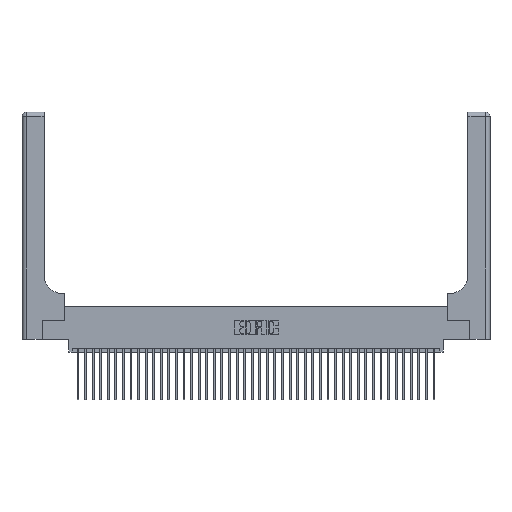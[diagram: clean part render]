
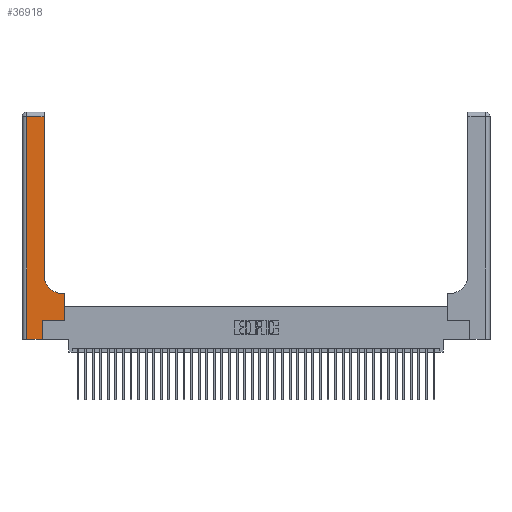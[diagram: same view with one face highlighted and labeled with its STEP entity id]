
A CAD part, top view. The second image highlights one B-rep face of the part: STEP entity #36918.
In plain terms, the highlighted planar face has unit normal (0, 0, 1).
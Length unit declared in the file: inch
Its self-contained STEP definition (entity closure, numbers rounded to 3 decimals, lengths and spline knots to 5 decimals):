
#201 = CARTESIAN_POINT ( 'NONE',  ( 0.2915, 0.85, 0.37 ) ) ;
#1006 = VECTOR ( 'NONE', #35913, 39.37008 ) ;
#1096 = DIRECTION ( 'NONE',  ( 1., 0., 0. ) ) ;
#3951 = CIRCLE ( 'NONE', #9672, 0.25 ) ;
#4097 = DIRECTION ( 'NONE',  ( 0., 0., -1. ) ) ;
#4598 = DIRECTION ( 'NONE',  ( -1., 0., 0. ) ) ;
#4820 = DIRECTION ( 'NONE',  ( 1., 0., 0. ) ) ;
#4827 = VECTOR ( 'NONE', #36877, 39.37008 ) ;
#6118 = VERTEX_POINT ( 'NONE', #28466 ) ;
#6372 = LINE ( 'NONE', #27816, #9430 ) ;
#6492 = CARTESIAN_POINT ( 'NONE',  ( 0., 0., 0.37 ) ) ;
#6857 = VECTOR ( 'NONE', #19501, 39.37008 ) ;
#6971 = AXIS2_PLACEMENT_3D ( 'NONE', #19197, #25766, #28636 ) ;
#7646 = CARTESIAN_POINT ( 'NONE',  ( 0.5415, 0.85, 0.37 ) ) ;
#8358 = ORIENTED_EDGE ( 'NONE', *, *, #18364, .T. ) ;
#8561 = DIRECTION ( 'NONE',  ( -1., 0., 0. ) ) ;
#8703 = VERTEX_POINT ( 'NONE', #28720 ) ;
#8882 = VERTEX_POINT ( 'NONE', #29566 ) ;
#9032 = VECTOR ( 'NONE', #8561, 39.37008 ) ;
#9430 = VECTOR ( 'NONE', #34122, 39.37008 ) ;
#9672 = AXIS2_PLACEMENT_3D ( 'NONE', #7646, #4097, #1096 ) ;
#9696 = PLANE ( 'NONE',  #6971 ) ;
#11051 = VECTOR ( 'NONE', #4820, 39.37008 ) ;
#11069 = LINE ( 'NONE', #24930, #9032 ) ;
#14468 = EDGE_LOOP ( 'NONE', ( #8358, #28727, #20410, #38125, #30006, #28920, #16696, #23089, #28937 ) ) ;
#16696 = ORIENTED_EDGE ( 'NONE', *, *, #33289, .T. ) ;
#17111 = CARTESIAN_POINT ( 'NONE',  ( 0.5585, 0.6, 0.37 ) ) ;
#17452 = VECTOR ( 'NONE', #23473, 39.37008 ) ;
#17636 = CARTESIAN_POINT ( 'NONE',  ( 0.5585, 0.25, 0.37 ) ) ;
#18219 = VERTEX_POINT ( 'NONE', #33816 ) ;
#18364 = EDGE_CURVE ( 'NONE', #40558, #8882, #31855, .T. ) ;
#18413 = EDGE_CURVE ( 'NONE', #29754, #8703, #22612, .T. ) ;
#19197 = CARTESIAN_POINT ( 'NONE',  ( 0., 3., 0.37 ) ) ;
#19319 = CARTESIAN_POINT ( 'NONE',  ( 0.2915, 3., 0.37 ) ) ;
#19471 = VERTEX_POINT ( 'NONE', #30650 ) ;
#19501 = DIRECTION ( 'NONE',  ( 1., 0., 0. ) ) ;
#19685 = LINE ( 'NONE', #33633, #11051 ) ;
#19807 = EDGE_CURVE ( 'NONE', #31629, #18219, #21995, .T. ) ;
#20410 = ORIENTED_EDGE ( 'NONE', *, *, #22743, .T. ) ;
#20805 = CARTESIAN_POINT ( 'NONE',  ( 0.2915, 0.6, 0.37 ) ) ;
#21995 = LINE ( 'NONE', #20805, #25570 ) ;
#22612 = LINE ( 'NONE', #6492, #6857 ) ;
#22743 = EDGE_CURVE ( 'NONE', #6118, #29754, #6372, .T. ) ;
#23089 = ORIENTED_EDGE ( 'NONE', *, *, #19807, .T. ) ;
#23473 = DIRECTION ( 'NONE',  ( 0., 1., 0. ) ) ;
#24388 = FACE_OUTER_BOUND ( 'NONE', #14468, .T. ) ;
#24930 = CARTESIAN_POINT ( 'NONE',  ( 0., 2.94, 0.37 ) ) ;
#24996 = CARTESIAN_POINT ( 'NONE',  ( 0.06, 0., 0.37 ) ) ;
#25439 = EDGE_CURVE ( 'NONE', #8703, #35197, #38944, .T. ) ;
#25570 = VECTOR ( 'NONE', #4598, 39.37008 ) ;
#25766 = DIRECTION ( 'NONE',  ( 0., 0., -1. ) ) ;
#27131 = CARTESIAN_POINT ( 'NONE',  ( 0.269, 0.25, 0.37 ) ) ;
#27816 = CARTESIAN_POINT ( 'NONE',  ( 0.06, 3., 0.37 ) ) ;
#28466 = CARTESIAN_POINT ( 'NONE',  ( 0.06, 2.94, 0.37 ) ) ;
#28636 = DIRECTION ( 'NONE',  ( -1., 0., 0. ) ) ;
#28720 = CARTESIAN_POINT ( 'NONE',  ( 0.269, 0., 0.37 ) ) ;
#28727 = ORIENTED_EDGE ( 'NONE', *, *, #37650, .T. ) ;
#28920 = ORIENTED_EDGE ( 'NONE', *, *, #29064, .T. ) ;
#28937 = ORIENTED_EDGE ( 'NONE', *, *, #34166, .T. ) ;
#29064 = EDGE_CURVE ( 'NONE', #35197, #19471, #19685, .T. ) ;
#29566 = CARTESIAN_POINT ( 'NONE',  ( 0.2915, 2.94, 0.37 ) ) ;
#29754 = VERTEX_POINT ( 'NONE', #24996 ) ;
#30006 = ORIENTED_EDGE ( 'NONE', *, *, #25439, .T. ) ;
#30650 = CARTESIAN_POINT ( 'NONE',  ( 0.5585, 0.25, 0.37 ) ) ;
#31629 = VERTEX_POINT ( 'NONE', #17111 ) ;
#31855 = LINE ( 'NONE', #19319, #4827 ) ;
#33051 = CARTESIAN_POINT ( 'NONE',  ( 0.269, 0., 0.37 ) ) ;
#33289 = EDGE_CURVE ( 'NONE', #19471, #31629, #38741, .T. ) ;
#33633 = CARTESIAN_POINT ( 'NONE',  ( 0.269, 0.25, 0.37 ) ) ;
#33816 = CARTESIAN_POINT ( 'NONE',  ( 0.5415, 0.6, 0.37 ) ) ;
#34122 = DIRECTION ( 'NONE',  ( 0., -1., 0. ) ) ;
#34166 = EDGE_CURVE ( 'NONE', #18219, #40558, #3951, .T. ) ;
#35197 = VERTEX_POINT ( 'NONE', #27131 ) ;
#35913 = DIRECTION ( 'NONE',  ( 0., 1., 0. ) ) ;
#36877 = DIRECTION ( 'NONE',  ( 0., 1., 0. ) ) ;
#36918 = ADVANCED_FACE ( 'NONE', ( #24388 ), #9696, .F. ) ;
#37650 = EDGE_CURVE ( 'NONE', #8882, #6118, #11069, .T. ) ;
#38125 = ORIENTED_EDGE ( 'NONE', *, *, #18413, .T. ) ;
#38741 = LINE ( 'NONE', #17636, #1006 ) ;
#38944 = LINE ( 'NONE', #33051, #17452 ) ;
#40558 = VERTEX_POINT ( 'NONE', #201 ) ;
